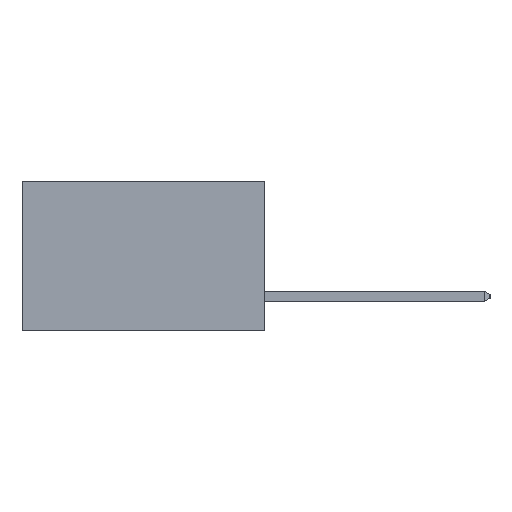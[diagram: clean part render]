
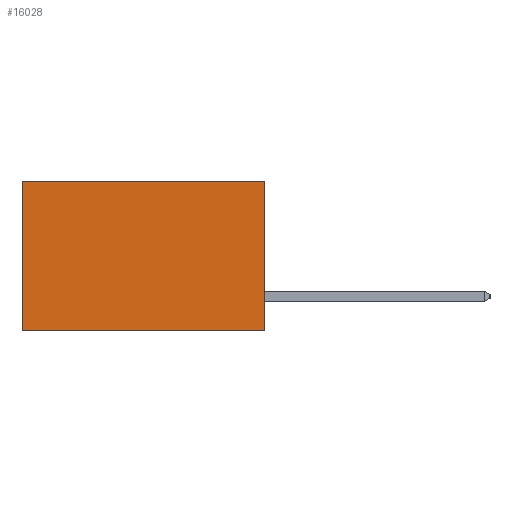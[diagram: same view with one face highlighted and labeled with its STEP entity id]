
A CAD part, left-side view. The second image highlights one B-rep face of the part: STEP entity #16028.
In plain terms, the highlighted planar face has unit normal (-1, 0, 0).
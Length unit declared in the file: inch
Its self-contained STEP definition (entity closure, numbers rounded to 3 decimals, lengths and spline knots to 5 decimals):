
#197 = DIRECTION ( 'NONE',  ( 0., 1., 0. ) ) ;
#304 = LINE ( 'NONE', #16166, #8495 ) ;
#933 = EDGE_CURVE ( 'NONE', #4599, #18633, #5190, .T. ) ;
#1052 = DIRECTION ( 'NONE',  ( 0., 1., 0. ) ) ;
#2045 = LINE ( 'NONE', #5777, #5863 ) ;
#3620 = CARTESIAN_POINT ( 'NONE',  ( 0.298, 0., 0. ) ) ;
#3696 = DIRECTION ( 'NONE',  ( 1., 0., 0. ) ) ;
#3928 = ORIENTED_EDGE ( 'NONE', *, *, #933, .F. ) ;
#4466 = CARTESIAN_POINT ( 'NONE',  ( 0.298, 0., -0.37 ) ) ;
#4599 = VERTEX_POINT ( 'NONE', #4466 ) ;
#4906 = VECTOR ( 'NONE', #1052, 39.37008 ) ;
#5190 = LINE ( 'NONE', #18268, #18724 ) ;
#5777 = CARTESIAN_POINT ( 'NONE',  ( 0.298, 0., 0. ) ) ;
#5863 = VECTOR ( 'NONE', #18807, 39.37008 ) ;
#8052 = DIRECTION ( 'NONE',  ( 0., 0., -1. ) ) ;
#8325 = ORIENTED_EDGE ( 'NONE', *, *, #11686, .T. ) ;
#8495 = VECTOR ( 'NONE', #8052, 39.37008 ) ;
#8717 = CARTESIAN_POINT ( 'NONE',  ( 0.298, 0.6, 0. ) ) ;
#8757 = LINE ( 'NONE', #17294, #4906 ) ;
#8769 = EDGE_LOOP ( 'NONE', ( #11335, #3928, #12452, #8325 ) ) ;
#11335 = ORIENTED_EDGE ( 'NONE', *, *, #20855, .T. ) ;
#11686 = EDGE_CURVE ( 'NONE', #13314, #19460, #8757, .T. ) ;
#12452 = ORIENTED_EDGE ( 'NONE', *, *, #18217, .F. ) ;
#13314 = VERTEX_POINT ( 'NONE', #3620 ) ;
#13475 = CARTESIAN_POINT ( 'NONE',  ( 0.298, 0., 0. ) ) ;
#15096 = DIRECTION ( 'NONE',  ( 0., 0., -1. ) ) ;
#15442 = AXIS2_PLACEMENT_3D ( 'NONE', #13475, #3696, #15096 ) ;
#16028 = ADVANCED_FACE ( 'NONE', ( #19690 ), #16649, .F. ) ;
#16166 = CARTESIAN_POINT ( 'NONE',  ( 0.298, 0.6, 0. ) ) ;
#16649 = PLANE ( 'NONE',  #15442 ) ;
#17294 = CARTESIAN_POINT ( 'NONE',  ( 0.298, 0., 0. ) ) ;
#18141 = CARTESIAN_POINT ( 'NONE',  ( 0.298, 0.6, -0.37 ) ) ;
#18217 = EDGE_CURVE ( 'NONE', #13314, #4599, #2045, .T. ) ;
#18268 = CARTESIAN_POINT ( 'NONE',  ( 0.298, 0., -0.37 ) ) ;
#18633 = VERTEX_POINT ( 'NONE', #18141 ) ;
#18724 = VECTOR ( 'NONE', #197, 39.37008 ) ;
#18807 = DIRECTION ( 'NONE',  ( 0., 0., -1. ) ) ;
#19460 = VERTEX_POINT ( 'NONE', #8717 ) ;
#19690 = FACE_OUTER_BOUND ( 'NONE', #8769, .T. ) ;
#20855 = EDGE_CURVE ( 'NONE', #19460, #18633, #304, .T. ) ;
